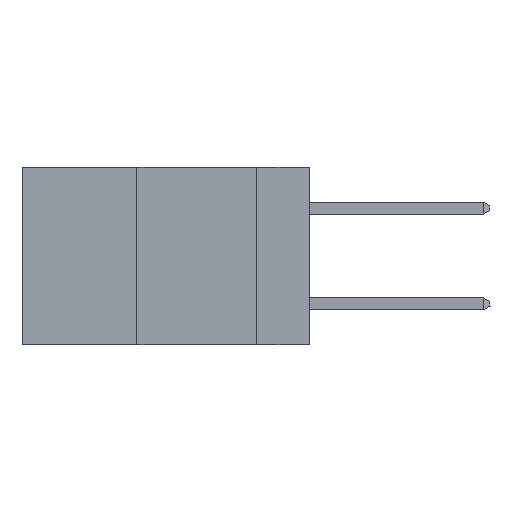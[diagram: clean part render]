
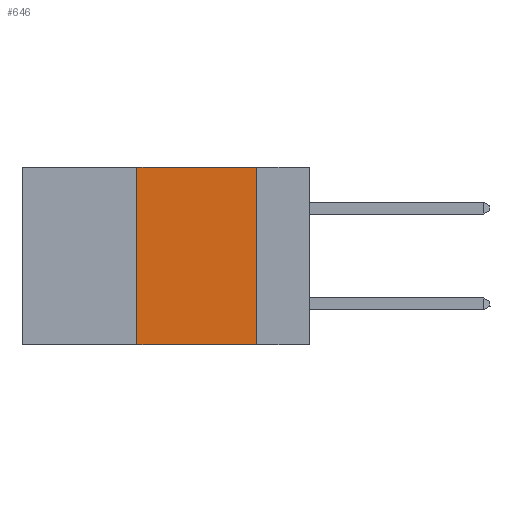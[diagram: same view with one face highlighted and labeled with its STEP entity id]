
A CAD part, left-side view. The second image highlights one B-rep face of the part: STEP entity #646.
In plain terms, the highlighted planar face has unit normal (-1, 0, 0).
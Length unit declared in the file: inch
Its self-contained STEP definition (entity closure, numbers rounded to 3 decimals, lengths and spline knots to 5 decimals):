
#646 = ADVANCED_FACE ( 'NONE', ( #25625 ), #5829, .F. ) ;
#1198 = VECTOR ( 'NONE', #2802, 39.37008 ) ;
#1983 = LINE ( 'NONE', #21802, #20522 ) ;
#2802 = DIRECTION ( 'NONE',  ( 0., 0., 1. ) ) ;
#3674 = ORIENTED_EDGE ( 'NONE', *, *, #23722, .F. ) ;
#4191 = EDGE_CURVE ( 'NONE', #12439, #8487, #1983, .T. ) ;
#4576 = CARTESIAN_POINT ( 'NONE',  ( 0., 0.36, 0. ) ) ;
#5829 = PLANE ( 'NONE',  #24511 ) ;
#6603 = LINE ( 'NONE', #10756, #1198 ) ;
#8487 = VERTEX_POINT ( 'NONE', #11517 ) ;
#8718 = VERTEX_POINT ( 'NONE', #4576 ) ;
#10318 = ORIENTED_EDGE ( 'NONE', *, *, #4191, .T. ) ;
#10756 = CARTESIAN_POINT ( 'NONE',  ( 0., 0.36, 0. ) ) ;
#11221 = DIRECTION ( 'NONE',  ( 0., 0., -1. ) ) ;
#11517 = CARTESIAN_POINT ( 'NONE',  ( 0., 0.11, -0.37 ) ) ;
#11766 = VECTOR ( 'NONE', #11221, 39.37008 ) ;
#12195 = EDGE_LOOP ( 'NONE', ( #24284, #13862, #3674, #10318 ) ) ;
#12439 = VERTEX_POINT ( 'NONE', #19313 ) ;
#12601 = VERTEX_POINT ( 'NONE', #13623 ) ;
#13623 = CARTESIAN_POINT ( 'NONE',  ( 0., 0.11, 0. ) ) ;
#13862 = ORIENTED_EDGE ( 'NONE', *, *, #15427, .F. ) ;
#13886 = DIRECTION ( 'NONE',  ( 0., -1., 0. ) ) ;
#14105 = EDGE_CURVE ( 'NONE', #12601, #8487, #19406, .T. ) ;
#14481 = LINE ( 'NONE', #16169, #20809 ) ;
#15427 = EDGE_CURVE ( 'NONE', #8718, #12601, #14481, .T. ) ;
#15630 = CARTESIAN_POINT ( 'NONE',  ( 0., 0.6, 0. ) ) ;
#16169 = CARTESIAN_POINT ( 'NONE',  ( 0., 0.6, 0. ) ) ;
#16552 = DIRECTION ( 'NONE',  ( 0., -1., 0. ) ) ;
#16856 = CARTESIAN_POINT ( 'NONE',  ( 0., 0.11, 0. ) ) ;
#19313 = CARTESIAN_POINT ( 'NONE',  ( 0., 0.36, -0.37 ) ) ;
#19406 = LINE ( 'NONE', #16856, #11766 ) ;
#19482 = DIRECTION ( 'NONE',  ( 0., 0., -1. ) ) ;
#20522 = VECTOR ( 'NONE', #13886, 39.37008 ) ;
#20809 = VECTOR ( 'NONE', #16552, 39.37008 ) ;
#21802 = CARTESIAN_POINT ( 'NONE',  ( 0., 0.6, -0.37 ) ) ;
#23672 = DIRECTION ( 'NONE',  ( 1., 0., 0. ) ) ;
#23722 = EDGE_CURVE ( 'NONE', #12439, #8718, #6603, .T. ) ;
#24284 = ORIENTED_EDGE ( 'NONE', *, *, #14105, .F. ) ;
#24511 = AXIS2_PLACEMENT_3D ( 'NONE', #15630, #23672, #19482 ) ;
#25625 = FACE_OUTER_BOUND ( 'NONE', #12195, .T. ) ;
